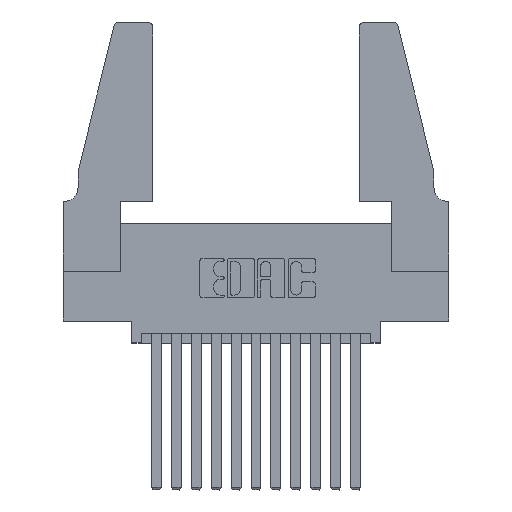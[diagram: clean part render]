
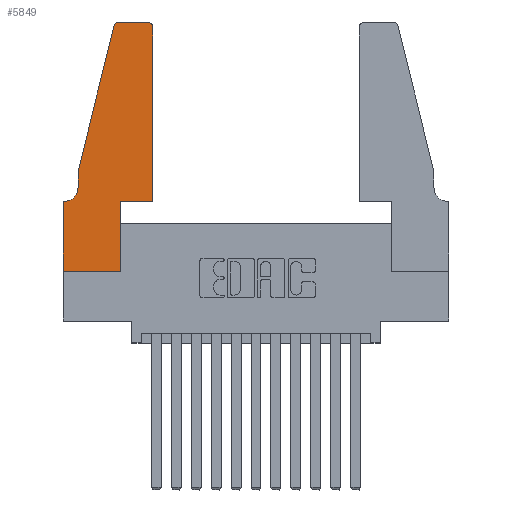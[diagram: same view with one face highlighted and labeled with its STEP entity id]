
A CAD part, top view. The second image highlights one B-rep face of the part: STEP entity #5849.
In plain terms, the highlighted planar face has unit normal (0, 0, 1).
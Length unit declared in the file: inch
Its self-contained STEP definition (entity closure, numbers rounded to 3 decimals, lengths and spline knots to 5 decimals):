
#23 = VERTEX_POINT ( 'NONE', #12874 ) ;
#59 = CARTESIAN_POINT ( 'NONE',  ( 0.4505, 0.35, 0.37 ) ) ;
#448 = ORIENTED_EDGE ( 'NONE', *, *, #10351, .T. ) ;
#821 = ORIENTED_EDGE ( 'NONE', *, *, #4459, .T. ) ;
#893 = EDGE_LOOP ( 'NONE', ( #11734, #9148, #12104, #9497, #448, #9867, #821, #13136, #1192, #4759, #7943, #1952 ) ) ;
#1014 = CARTESIAN_POINT ( 'NONE',  ( 0., 0., 0.37 ) ) ;
#1192 = ORIENTED_EDGE ( 'NONE', *, *, #4213, .T. ) ;
#1456 = CARTESIAN_POINT ( 'NONE',  ( 0., 0., 0.37 ) ) ;
#1920 = AXIS2_PLACEMENT_3D ( 'NONE', #11785, #4931, #12896 ) ;
#1921 = CARTESIAN_POINT ( 'NONE',  ( 0., 0.35, 0.37 ) ) ;
#1952 = ORIENTED_EDGE ( 'NONE', *, *, #7624, .T. ) ;
#2121 = VERTEX_POINT ( 'NONE', #5470 ) ;
#2131 = VERTEX_POINT ( 'NONE', #5435 ) ;
#2195 = DIRECTION ( 'NONE',  ( 0., -1., 0. ) ) ;
#2806 = VERTEX_POINT ( 'NONE', #3959 ) ;
#3075 = LINE ( 'NONE', #3130, #5915 ) ;
#3130 = CARTESIAN_POINT ( 'NONE',  ( 0.2605, 1.25, 0.37 ) ) ;
#3235 = VERTEX_POINT ( 'NONE', #1921 ) ;
#3292 = CIRCLE ( 'NONE', #14230, 0.03 ) ;
#3693 = EDGE_CURVE ( 'NONE', #23, #2806, #6978, .T. ) ;
#3914 = CARTESIAN_POINT ( 'NONE',  ( 0.2865, 0., 0.37 ) ) ;
#3919 = CARTESIAN_POINT ( 'NONE',  ( 0., 0.35, 0.37 ) ) ;
#3939 = LINE ( 'NONE', #5670, #9807 ) ;
#3959 = CARTESIAN_POINT ( 'NONE',  ( 0.4505, 1.22, 0.37 ) ) ;
#4213 = EDGE_CURVE ( 'NONE', #7555, #14009, #10327, .T. ) ;
#4459 = EDGE_CURVE ( 'NONE', #3235, #4853, #10151, .T. ) ;
#4482 = DIRECTION ( 'NONE',  ( -1., 0., 0. ) ) ;
#4611 = CARTESIAN_POINT ( 'NONE',  ( 0.0755, 0.5, 0.37 ) ) ;
#4759 = ORIENTED_EDGE ( 'NONE', *, *, #13145, .T. ) ;
#4853 = VERTEX_POINT ( 'NONE', #1014 ) ;
#4858 = DIRECTION ( 'NONE',  ( 0., 0., 1. ) ) ;
#4924 = EDGE_CURVE ( 'NONE', #2121, #12853, #9784, .T. ) ;
#4931 = DIRECTION ( 'NONE',  ( 0., 0., -1. ) ) ;
#5148 = DIRECTION ( 'NONE',  ( 0., 0., 1. ) ) ;
#5435 = CARTESIAN_POINT ( 'NONE',  ( 0.284, 1.25, 0.37 ) ) ;
#5470 = CARTESIAN_POINT ( 'NONE',  ( 0.25487, 1.22718, 0.37 ) ) ;
#5670 = CARTESIAN_POINT ( 'NONE',  ( 0., 0., 0.37 ) ) ;
#5849 = ADVANCED_FACE ( 'NONE', ( #13706 ), #10867, .T. ) ;
#5915 = VECTOR ( 'NONE', #13468, 39.37008 ) ;
#6002 = DIRECTION ( 'NONE',  ( 0., 1., 0. ) ) ;
#6403 = VECTOR ( 'NONE', #4482, 39.37008 ) ;
#6454 = CARTESIAN_POINT ( 'NONE',  ( 0.4205, 1.22, 0.37 ) ) ;
#6760 = VECTOR ( 'NONE', #14919, 39.37008 ) ;
#6777 = VECTOR ( 'NONE', #11903, 39.37008 ) ;
#6788 = LINE ( 'NONE', #13559, #6403 ) ;
#6882 = DIRECTION ( 'NONE',  ( 1., 0., 0. ) ) ;
#6978 = LINE ( 'NONE', #59, #12554 ) ;
#7031 = DIRECTION ( 'NONE',  ( 0., 1., 0. ) ) ;
#7462 = CARTESIAN_POINT ( 'NONE',  ( 0.2865, 0.35, 0.37 ) ) ;
#7555 = VERTEX_POINT ( 'NONE', #3914 ) ;
#7624 = EDGE_CURVE ( 'NONE', #2806, #13049, #12842, .T. ) ;
#7673 = DIRECTION ( 'NONE',  ( 1., 0., 0. ) ) ;
#7943 = ORIENTED_EDGE ( 'NONE', *, *, #3693, .T. ) ;
#8090 = VECTOR ( 'NONE', #13504, 39.37008 ) ;
#8098 = EDGE_CURVE ( 'NONE', #2131, #2121, #3292, .T. ) ;
#8464 = AXIS2_PLACEMENT_3D ( 'NONE', #3919, #5148, #13086 ) ;
#9137 = EDGE_CURVE ( 'NONE', #13049, #2131, #3075, .T. ) ;
#9148 = ORIENTED_EDGE ( 'NONE', *, *, #8098, .T. ) ;
#9287 = EDGE_CURVE ( 'NONE', #12853, #11452, #13138, .T. ) ;
#9497 = ORIENTED_EDGE ( 'NONE', *, *, #9287, .T. ) ;
#9784 = LINE ( 'NONE', #10513, #6760 ) ;
#9807 = VECTOR ( 'NONE', #6882, 39.37008 ) ;
#9867 = ORIENTED_EDGE ( 'NONE', *, *, #14397, .T. ) ;
#10151 = LINE ( 'NONE', #1456, #6777 ) ;
#10193 = CARTESIAN_POINT ( 'NONE',  ( 0.4505, 0.35, 0.37 ) ) ;
#10276 = VERTEX_POINT ( 'NONE', #10938 ) ;
#10327 = LINE ( 'NONE', #14618, #12894 ) ;
#10351 = EDGE_CURVE ( 'NONE', #11452, #10276, #12923, .T. ) ;
#10513 = CARTESIAN_POINT ( 'NONE',  ( 0.0755, 0.5, 0.37 ) ) ;
#10616 = CARTESIAN_POINT ( 'NONE',  ( 0.0755, 0.42, 0.37 ) ) ;
#10867 = PLANE ( 'NONE',  #8464 ) ;
#10938 = CARTESIAN_POINT ( 'NONE',  ( 0.0055, 0.35, 0.37 ) ) ;
#11452 = VERTEX_POINT ( 'NONE', #10616 ) ;
#11697 = CARTESIAN_POINT ( 'NONE',  ( 0.284, 1.22, 0.37 ) ) ;
#11734 = ORIENTED_EDGE ( 'NONE', *, *, #9137, .T. ) ;
#11785 = CARTESIAN_POINT ( 'NONE',  ( 0.0055, 0.42, 0.37 ) ) ;
#11903 = DIRECTION ( 'NONE',  ( 0., -1., 0. ) ) ;
#12104 = ORIENTED_EDGE ( 'NONE', *, *, #4924, .T. ) ;
#12554 = VECTOR ( 'NONE', #6002, 39.37008 ) ;
#12780 = VECTOR ( 'NONE', #2195, 39.37008 ) ;
#12817 = DIRECTION ( 'NONE',  ( 1., 0., 0. ) ) ;
#12842 = CIRCLE ( 'NONE', #13014, 0.03 ) ;
#12853 = VERTEX_POINT ( 'NONE', #14138 ) ;
#12874 = CARTESIAN_POINT ( 'NONE',  ( 0.4505, 0.35, 0.37 ) ) ;
#12894 = VECTOR ( 'NONE', #7031, 39.37008 ) ;
#12896 = DIRECTION ( 'NONE',  ( -1., 0., 0. ) ) ;
#12923 = CIRCLE ( 'NONE', #1920, 0.07 ) ;
#13014 = AXIS2_PLACEMENT_3D ( 'NONE', #6454, #14293, #7673 ) ;
#13049 = VERTEX_POINT ( 'NONE', #14422 ) ;
#13086 = DIRECTION ( 'NONE',  ( 1., 0., 0. ) ) ;
#13136 = ORIENTED_EDGE ( 'NONE', *, *, #14350, .T. ) ;
#13138 = LINE ( 'NONE', #4611, #12780 ) ;
#13145 = EDGE_CURVE ( 'NONE', #14009, #23, #13963, .T. ) ;
#13468 = DIRECTION ( 'NONE',  ( -1., 0., 0. ) ) ;
#13504 = DIRECTION ( 'NONE',  ( 1., 0., 0. ) ) ;
#13559 = CARTESIAN_POINT ( 'NONE',  ( 0.0755, 0.35, 0.37 ) ) ;
#13706 = FACE_OUTER_BOUND ( 'NONE', #893, .T. ) ;
#13963 = LINE ( 'NONE', #10193, #8090 ) ;
#14009 = VERTEX_POINT ( 'NONE', #7462 ) ;
#14138 = CARTESIAN_POINT ( 'NONE',  ( 0.0755, 0.5, 0.37 ) ) ;
#14230 = AXIS2_PLACEMENT_3D ( 'NONE', #11697, #4858, #12817 ) ;
#14293 = DIRECTION ( 'NONE',  ( 0., 0., 1. ) ) ;
#14350 = EDGE_CURVE ( 'NONE', #4853, #7555, #3939, .T. ) ;
#14397 = EDGE_CURVE ( 'NONE', #10276, #3235, #6788, .T. ) ;
#14422 = CARTESIAN_POINT ( 'NONE',  ( 0.4205, 1.25, 0.37 ) ) ;
#14618 = CARTESIAN_POINT ( 'NONE',  ( 0.2865, 0.35, 0.37 ) ) ;
#14919 = DIRECTION ( 'NONE',  ( -0.239, -0.971, 0. ) ) ;
